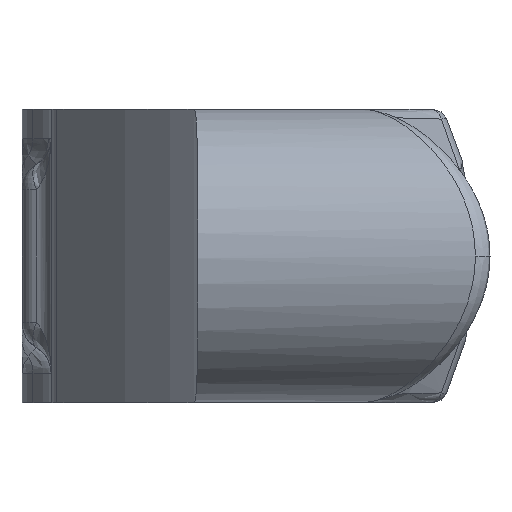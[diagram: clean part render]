
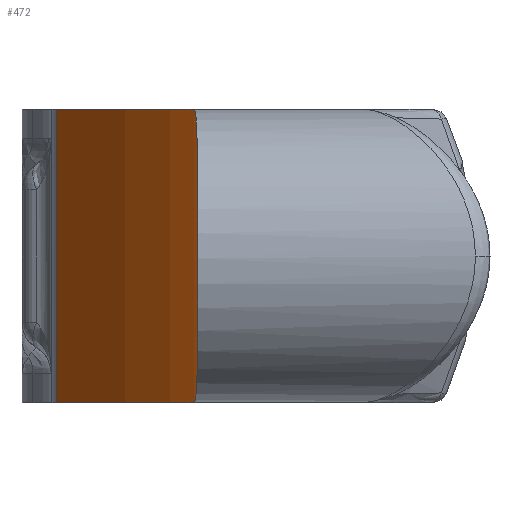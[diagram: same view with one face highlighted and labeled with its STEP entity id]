
A CAD part, front view. The second image highlights one B-rep face of the part: STEP entity #472.
In plain terms, the highlighted cylindrical face has radius 125 mm (diameter 250 mm), a partial arc.
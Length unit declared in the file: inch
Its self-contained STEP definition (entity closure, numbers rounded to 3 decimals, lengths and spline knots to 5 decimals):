
#60 = CARTESIAN_POINT ( 'NONE',  ( 1.71365, -3.29228, 0.3937 ) ) ;
#98 = CARTESIAN_POINT ( 'NONE',  ( 6.63263, -3.14251, 0.0125 ) ) ;
#114 = CARTESIAN_POINT ( 'NONE',  ( 6.63486, -3.27001, 0.20985 ) ) ;
#120 = CARTESIAN_POINT ( 'NONE',  ( 1.71365, -3.29228, 0. ) ) ;
#126 = CARTESIAN_POINT ( 'NONE',  ( 6.63315, -3.16046, 0.37375 ) ) ;
#197 = CARTESIAN_POINT ( 'NONE',  ( 1.71365, -3.29228, 0.3937 ) ) ;
#320 = DIRECTION ( 'NONE',  ( 1., 0., 0. ) ) ;
#340 = CARTESIAN_POINT ( 'NONE',  ( 6.63003, -3.07316, 0. ) ) ;
#355 = CARTESIAN_POINT ( 'NONE',  ( 6.63344, -3.17168, 0.02594 ) ) ;
#364 = CARTESIAN_POINT ( 'NONE',  ( 6.63483, -3.26499, 0.2415 ) ) ;
#370 = DIRECTION ( 'NONE',  ( 1., 0., 0. ) ) ;
#377 = CARTESIAN_POINT ( 'NONE',  ( 6.63206, -3.12442, 0.38735 ) ) ;
#414 = CIRCLE ( 'NONE', #2512, 4.92126 ) ;
#465 = ORIENTED_EDGE ( 'NONE', *, *, #1631, .F. ) ;
#472 = ADVANCED_FACE ( 'NONE', ( #1924 ), #1851, .F. ) ;
#572 = CIRCLE ( 'NONE', #1184, 4.92126 ) ;
#597 = CARTESIAN_POINT ( 'NONE',  ( 6.63411, -3.2032, 0.04851 ) ) ;
#611 = CARTESIAN_POINT ( 'NONE',  ( 6.6348, -3.25969, 0.26009 ) ) ;
#624 = CARTESIAN_POINT ( 'NONE',  ( 6.6306, -3.08615, 0.3937 ) ) ;
#845 = CARTESIAN_POINT ( 'NONE',  ( 6.63451, -3.22952, 0.07656 ) ) ;
#856 = CARTESIAN_POINT ( 'NONE',  ( 6.63473, -3.25009, 0.28411 ) ) ;
#1033 = B_SPLINE_CURVE_WITH_KNOTS ( 'NONE', 3,
 ( #340, #2188, #2653, #1282, #2876, #1518, #98, #1745, #355, #1970, #597, #2200, #845, #2432, #1068, #2670, #1295, #2886, #1529, #114, #1758, #364, #1986, #611, #2209, #856, #2445, #1081, #2681, #1308, #2894, #1541, #126, #1770, #377, #1997, #624, #2219 ),
 .UNSPECIFIED., .F., .F.,
 ( 4, 2, 2, 2, 2, 2, 2, 2, 2, 2, 2, 2, 2, 2, 2, 2, 2, 2, 4 ),
 ( 0., 0.00098, 0.00146, 0.00195, 0.00293, 0.00391, 0.00488, 0.00586, 0.00684, 0.00781, 0.00879, 0.00928, 0.00977, 0.01074, 0.01172, 0.0127, 0.01367, 0.01465, 0.01563 ),
 .UNSPECIFIED. ) ;
#1068 = CARTESIAN_POINT ( 'NONE',  ( 6.63473, -3.25004, 0.10951 ) ) ;
#1070 = CARTESIAN_POINT ( 'NONE',  ( 6.63003, -3.07316, 0.3937 ) ) ;
#1081 = CARTESIAN_POINT ( 'NONE',  ( 6.63451, -3.22977, 0.31681 ) ) ;
#1088 = VERTEX_POINT ( 'NONE', #1070 ) ;
#1096 = ORIENTED_EDGE ( 'NONE', *, *, #1628, .F. ) ;
#1111 = VECTOR ( 'NONE', #2780, 39.37008 ) ;
#1126 = ORIENTED_EDGE ( 'NONE', *, *, #1171, .F. ) ;
#1171 = EDGE_CURVE ( 'NONE', #1527, #2119, #572, .T. ) ;
#1184 = AXIS2_PLACEMENT_3D ( 'NONE', #120, #1762, #370 ) ;
#1282 = CARTESIAN_POINT ( 'NONE',  ( 6.63182, -3.11778, 0.00501 ) ) ;
#1295 = CARTESIAN_POINT ( 'NONE',  ( 6.63482, -3.26366, 0.14556 ) ) ;
#1308 = CARTESIAN_POINT ( 'NONE',  ( 6.63411, -3.20331, 0.3451 ) ) ;
#1395 = CARTESIAN_POINT ( 'NONE',  ( 6.63003, -3.07316, 0. ) ) ;
#1482 = EDGE_LOOP ( 'NONE', ( #1126, #2161, #1096, #465 ) ) ;
#1518 = CARTESIAN_POINT ( 'NONE',  ( 6.63244, -3.13636, 0.01031 ) ) ;
#1527 = VERTEX_POINT ( 'NONE', #1395 ) ;
#1529 = CARTESIAN_POINT ( 'NONE',  ( 6.63486, -3.27001, 0.18385 ) ) ;
#1541 = CARTESIAN_POINT ( 'NONE',  ( 6.63345, -3.17191, 0.36763 ) ) ;
#1628 = EDGE_CURVE ( 'NONE', #2868, #1088, #414, .T. ) ;
#1631 = EDGE_CURVE ( 'NONE', #2119, #2868, #2854, .T. ) ;
#1712 = DIRECTION ( 'NONE',  ( 0., 0., -1. ) ) ;
#1745 = CARTESIAN_POINT ( 'NONE',  ( 6.63315, -3.16038, 0.0199 ) ) ;
#1758 = CARTESIAN_POINT ( 'NONE',  ( 6.63485, -3.26874, 0.22263 ) ) ;
#1762 = DIRECTION ( 'NONE',  ( 0., 0., 1. ) ) ;
#1770 = CARTESIAN_POINT ( 'NONE',  ( 6.63246, -3.13679, 0.38357 ) ) ;
#1828 = DIRECTION ( 'NONE',  ( 0., 0., 1. ) ) ;
#1834 = CARTESIAN_POINT ( 'NONE',  ( 6.44558, -1.94039, 0. ) ) ;
#1851 = CYLINDRICAL_SURFACE ( 'NONE', #2729, 4.92126 ) ;
#1895 = EDGE_CURVE ( 'NONE', #1527, #1088, #1033, .T. ) ;
#1924 = FACE_OUTER_BOUND ( 'NONE', #1482, .T. ) ;
#1970 = CARTESIAN_POINT ( 'NONE',  ( 6.63392, -3.19307, 0.04021 ) ) ;
#1986 = CARTESIAN_POINT ( 'NONE',  ( 6.63482, -3.26343, 0.24773 ) ) ;
#1997 = CARTESIAN_POINT ( 'NONE',  ( 6.63113, -3.099, 0.39243 ) ) ;
#2064 = DIRECTION ( 'NONE',  ( 1., 0., 0. ) ) ;
#2119 = VERTEX_POINT ( 'NONE', #1834 ) ;
#2161 = ORIENTED_EDGE ( 'NONE', *, *, #1895, .T. ) ;
#2188 = CARTESIAN_POINT ( 'NONE',  ( 6.6306, -3.08615, 0. ) ) ;
#2200 = CARTESIAN_POINT ( 'NONE',  ( 6.6344, -3.22137, 0.06666 ) ) ;
#2209 = CARTESIAN_POINT ( 'NONE',  ( 6.63478, -3.25749, 0.26624 ) ) ;
#2219 = CARTESIAN_POINT ( 'NONE',  ( 6.63003, -3.07316, 0.3937 ) ) ;
#2432 = CARTESIAN_POINT ( 'NONE',  ( 6.63467, -3.24392, 0.09806 ) ) ;
#2445 = CARTESIAN_POINT ( 'NONE',  ( 6.63468, -3.24404, 0.29542 ) ) ;
#2477 = CARTESIAN_POINT ( 'NONE',  ( 6.44558, -1.94039, 0.3937 ) ) ;
#2512 = AXIS2_PLACEMENT_3D ( 'NONE', #60, #1712, #320 ) ;
#2544 = CARTESIAN_POINT ( 'NONE',  ( 6.44558, -1.94039, 0.3937 ) ) ;
#2653 = CARTESIAN_POINT ( 'NONE',  ( 6.63112, -3.09892, 0.00127 ) ) ;
#2670 = CARTESIAN_POINT ( 'NONE',  ( 6.6348, -3.25987, 0.13318 ) ) ;
#2681 = CARTESIAN_POINT ( 'NONE',  ( 6.63441, -3.22146, 0.32694 ) ) ;
#2729 = AXIS2_PLACEMENT_3D ( 'NONE', #197, #1828, #2064 ) ;
#2780 = DIRECTION ( 'NONE',  ( 0., 0., 1. ) ) ;
#2854 = LINE ( 'NONE', #2544, #1111 ) ;
#2868 = VERTEX_POINT ( 'NONE', #2477 ) ;
#2876 = CARTESIAN_POINT ( 'NONE',  ( 6.63203, -3.12401, 0.00657 ) ) ;
#2886 = CARTESIAN_POINT ( 'NONE',  ( 6.63485, -3.26874, 0.17099 ) ) ;
#2894 = CARTESIAN_POINT ( 'NONE',  ( 6.63392, -3.19341, 0.35324 ) ) ;
